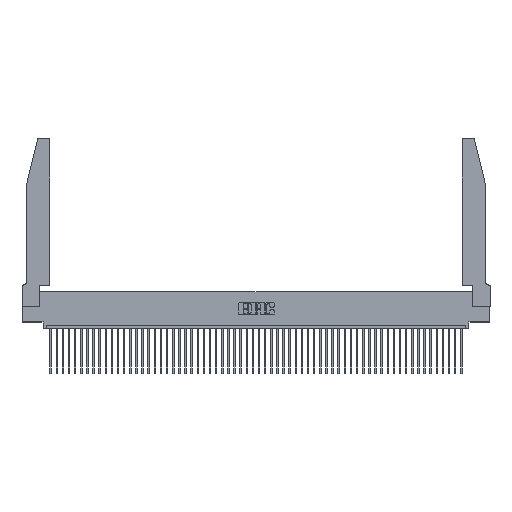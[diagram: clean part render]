
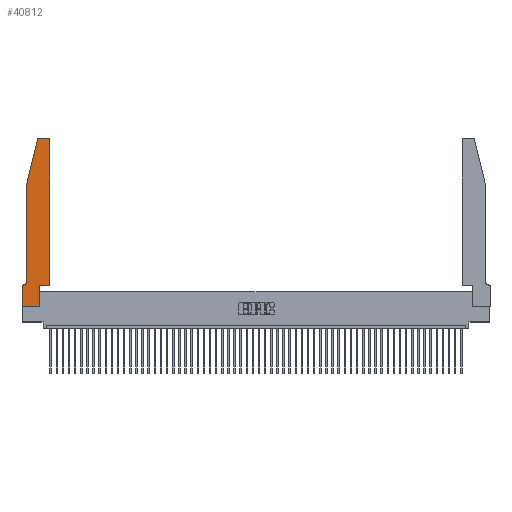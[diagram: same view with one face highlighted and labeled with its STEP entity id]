
A CAD part, top view. The second image highlights one B-rep face of the part: STEP entity #40812.
In plain terms, the highlighted planar face has unit normal (0, 0, 1).
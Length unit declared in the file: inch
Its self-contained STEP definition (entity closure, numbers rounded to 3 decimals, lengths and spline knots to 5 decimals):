
#1354 = VECTOR ( 'NONE', #10473, 39.37008 ) ;
#2323 = CARTESIAN_POINT ( 'NONE',  ( 0.0755, 2., 0.37 ) ) ;
#2703 = CARTESIAN_POINT ( 'NONE',  ( 0.2865, 0.35, 0.37 ) ) ;
#3601 = VECTOR ( 'NONE', #6423, 39.37008 ) ;
#3734 = CARTESIAN_POINT ( 'NONE',  ( 0., 0.35, 0.37 ) ) ;
#3750 = CARTESIAN_POINT ( 'NONE',  ( 0.4205, 2.72, 0.37 ) ) ;
#4453 = DIRECTION ( 'NONE',  ( 1., 0., 0. ) ) ;
#4949 = VERTEX_POINT ( 'NONE', #31778 ) ;
#5550 = LINE ( 'NONE', #20852, #41772 ) ;
#6319 = CARTESIAN_POINT ( 'NONE',  ( 0.2865, 0., 0.37 ) ) ;
#6423 = DIRECTION ( 'NONE',  ( 0., -1., 0. ) ) ;
#6706 = CARTESIAN_POINT ( 'NONE',  ( 0.4505, 0.35, 0.37 ) ) ;
#6723 = CARTESIAN_POINT ( 'NONE',  ( 0.4505, 0.35, 0.37 ) ) ;
#7171 = LINE ( 'NONE', #6706, #23079 ) ;
#7395 = CARTESIAN_POINT ( 'NONE',  ( 0., 0., 0.37 ) ) ;
#7441 = EDGE_CURVE ( 'NONE', #4949, #41382, #37669, .T. ) ;
#7688 = VECTOR ( 'NONE', #4453, 39.37008 ) ;
#8226 = VECTOR ( 'NONE', #47324, 39.37008 ) ;
#8523 = EDGE_LOOP ( 'NONE', ( #13742, #41669, #34876, #35065, #13721, #44714, #24916, #38572, #35421, #42227, #13220, #41159 ) ) ;
#9001 = CARTESIAN_POINT ( 'NONE',  ( 0.284, 2.72, 0.37 ) ) ;
#10322 = VERTEX_POINT ( 'NONE', #50298 ) ;
#10473 = DIRECTION ( 'NONE',  ( -0.239, -0.971, 0. ) ) ;
#12794 = DIRECTION ( 'NONE',  ( 1., 0., 0. ) ) ;
#13220 = ORIENTED_EDGE ( 'NONE', *, *, #40247, .T. ) ;
#13328 = CARTESIAN_POINT ( 'NONE',  ( 0.0755, 0.42, 0.37 ) ) ;
#13721 = ORIENTED_EDGE ( 'NONE', *, *, #45785, .T. ) ;
#13742 = ORIENTED_EDGE ( 'NONE', *, *, #16454, .T. ) ;
#14516 = VERTEX_POINT ( 'NONE', #13328 ) ;
#15256 = LINE ( 'NONE', #24059, #15840 ) ;
#15402 = CIRCLE ( 'NONE', #16373, 0.07 ) ;
#15546 = VERTEX_POINT ( 'NONE', #28974 ) ;
#15840 = VECTOR ( 'NONE', #39931, 39.37008 ) ;
#16373 = AXIS2_PLACEMENT_3D ( 'NONE', #40748, #32849, #49201 ) ;
#16454 = EDGE_CURVE ( 'NONE', #35767, #42054, #33335, .T. ) ;
#16942 = EDGE_CURVE ( 'NONE', #15546, #35767, #25626, .T. ) ;
#17026 = DIRECTION ( 'NONE',  ( -1., 0., 0. ) ) ;
#20782 = VERTEX_POINT ( 'NONE', #6319 ) ;
#20852 = CARTESIAN_POINT ( 'NONE',  ( 0.0755, 0.35, 0.37 ) ) ;
#21171 = VECTOR ( 'NONE', #17026, 39.37008 ) ;
#22696 = CARTESIAN_POINT ( 'NONE',  ( 0., 0., 0.37 ) ) ;
#23079 = VECTOR ( 'NONE', #23274, 39.37008 ) ;
#23250 = EDGE_CURVE ( 'NONE', #50349, #35318, #37360, .T. ) ;
#23274 = DIRECTION ( 'NONE',  ( 1., 0., 0. ) ) ;
#24059 = CARTESIAN_POINT ( 'NONE',  ( 0.4505, 0.35, 0.37 ) ) ;
#24070 = DIRECTION ( 'NONE',  ( 0., 0., 1. ) ) ;
#24382 = AXIS2_PLACEMENT_3D ( 'NONE', #3750, #24070, #44392 ) ;
#24602 = LINE ( 'NONE', #2323, #3601 ) ;
#24916 = ORIENTED_EDGE ( 'NONE', *, *, #23250, .T. ) ;
#25626 = CIRCLE ( 'NONE', #24382, 0.03 ) ;
#26015 = EDGE_CURVE ( 'NONE', #20782, #45784, #29677, .T. ) ;
#26155 = DIRECTION ( 'NONE',  ( 0., 0., 1. ) ) ;
#27094 = CARTESIAN_POINT ( 'NONE',  ( 0.0755, 2., 0.37 ) ) ;
#28974 = CARTESIAN_POINT ( 'NONE',  ( 0.4505, 2.72, 0.37 ) ) ;
#29064 = CARTESIAN_POINT ( 'NONE',  ( 0.2865, 0.35, 0.37 ) ) ;
#29205 = CARTESIAN_POINT ( 'NONE',  ( 0., 0.35, 0.37 ) ) ;
#29212 = CARTESIAN_POINT ( 'NONE',  ( 0.284, 2.75, 0.37 ) ) ;
#29677 = LINE ( 'NONE', #2703, #34428 ) ;
#31778 = CARTESIAN_POINT ( 'NONE',  ( 0.25487, 2.72718, 0.37 ) ) ;
#32849 = DIRECTION ( 'NONE',  ( 0., 0., -1. ) ) ;
#32901 = CIRCLE ( 'NONE', #45033, 0.03 ) ;
#32974 = PLANE ( 'NONE',  #45979 ) ;
#33129 = DIRECTION ( 'NONE',  ( 0., 0., 1. ) ) ;
#33335 = LINE ( 'NONE', #38141, #21171 ) ;
#34428 = VECTOR ( 'NONE', #36163, 39.37008 ) ;
#34876 = ORIENTED_EDGE ( 'NONE', *, *, #7441, .T. ) ;
#35065 = ORIENTED_EDGE ( 'NONE', *, *, #49605, .T. ) ;
#35318 = VERTEX_POINT ( 'NONE', #7395 ) ;
#35421 = ORIENTED_EDGE ( 'NONE', *, *, #26015, .T. ) ;
#35538 = FACE_OUTER_BOUND ( 'NONE', #8523, .T. ) ;
#35767 = VERTEX_POINT ( 'NONE', #37415 ) ;
#36163 = DIRECTION ( 'NONE',  ( 0., 1., 0. ) ) ;
#36338 = VERTEX_POINT ( 'NONE', #6723 ) ;
#37360 = LINE ( 'NONE', #22696, #8226 ) ;
#37415 = CARTESIAN_POINT ( 'NONE',  ( 0.4205, 2.75, 0.37 ) ) ;
#37439 = CARTESIAN_POINT ( 'NONE',  ( 0., 0., 0.37 ) ) ;
#37669 = LINE ( 'NONE', #27094, #1354 ) ;
#37810 = DIRECTION ( 'NONE',  ( 1., 0., 0. ) ) ;
#38126 = LINE ( 'NONE', #37439, #7688 ) ;
#38141 = CARTESIAN_POINT ( 'NONE',  ( 0.2605, 2.75, 0.37 ) ) ;
#38572 = ORIENTED_EDGE ( 'NONE', *, *, #46462, .T. ) ;
#39931 = DIRECTION ( 'NONE',  ( 0., 1., 0. ) ) ;
#40247 = EDGE_CURVE ( 'NONE', #36338, #15546, #15256, .T. ) ;
#40726 = EDGE_CURVE ( 'NONE', #10322, #50349, #5550, .T. ) ;
#40748 = CARTESIAN_POINT ( 'NONE',  ( 0.0055, 0.42, 0.37 ) ) ;
#40812 = ADVANCED_FACE ( 'NONE', ( #35538 ), #32974, .T. ) ;
#41159 = ORIENTED_EDGE ( 'NONE', *, *, #16942, .T. ) ;
#41382 = VERTEX_POINT ( 'NONE', #47267 ) ;
#41669 = ORIENTED_EDGE ( 'NONE', *, *, #49189, .T. ) ;
#41772 = VECTOR ( 'NONE', #49483, 39.37008 ) ;
#42054 = VERTEX_POINT ( 'NONE', #29212 ) ;
#42227 = ORIENTED_EDGE ( 'NONE', *, *, #45545, .T. ) ;
#44392 = DIRECTION ( 'NONE',  ( 1., 0., 0. ) ) ;
#44714 = ORIENTED_EDGE ( 'NONE', *, *, #40726, .T. ) ;
#45033 = AXIS2_PLACEMENT_3D ( 'NONE', #9001, #26155, #37810 ) ;
#45545 = EDGE_CURVE ( 'NONE', #45784, #36338, #7171, .T. ) ;
#45784 = VERTEX_POINT ( 'NONE', #29064 ) ;
#45785 = EDGE_CURVE ( 'NONE', #14516, #10322, #15402, .T. ) ;
#45979 = AXIS2_PLACEMENT_3D ( 'NONE', #29205, #33129, #12794 ) ;
#46462 = EDGE_CURVE ( 'NONE', #35318, #20782, #38126, .T. ) ;
#47267 = CARTESIAN_POINT ( 'NONE',  ( 0.0755, 2., 0.37 ) ) ;
#47324 = DIRECTION ( 'NONE',  ( 0., -1., 0. ) ) ;
#49189 = EDGE_CURVE ( 'NONE', #42054, #4949, #32901, .T. ) ;
#49201 = DIRECTION ( 'NONE',  ( -1., 0., 0. ) ) ;
#49483 = DIRECTION ( 'NONE',  ( -1., 0., 0. ) ) ;
#49605 = EDGE_CURVE ( 'NONE', #41382, #14516, #24602, .T. ) ;
#50298 = CARTESIAN_POINT ( 'NONE',  ( 0.0055, 0.35, 0.37 ) ) ;
#50349 = VERTEX_POINT ( 'NONE', #3734 ) ;
